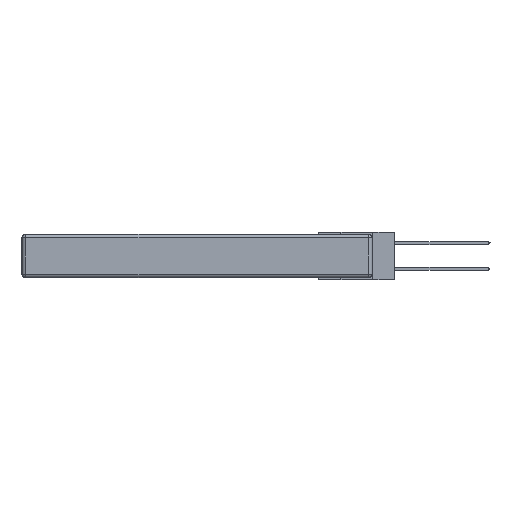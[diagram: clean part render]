
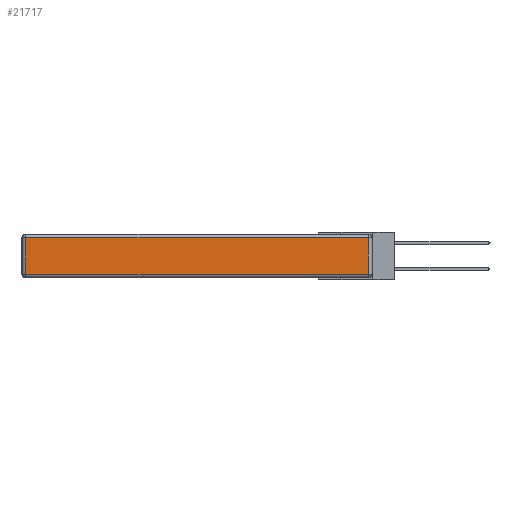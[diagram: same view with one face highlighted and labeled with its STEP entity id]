
A CAD part, left-side view. The second image highlights one B-rep face of the part: STEP entity #21717.
In plain terms, the highlighted planar face has unit normal (-1, 0, 0).
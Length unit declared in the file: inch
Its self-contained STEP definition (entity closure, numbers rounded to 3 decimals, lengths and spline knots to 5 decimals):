
#26 = DIRECTION ( 'NONE',  ( 0., 0., -1. ) ) ;
#100 = CARTESIAN_POINT ( 'NONE',  ( 0., 2.72, -0.313 ) ) ;
#958 = LINE ( 'NONE', #12153, #4760 ) ;
#1406 = ORIENTED_EDGE ( 'NONE', *, *, #11649, .T. ) ;
#1409 = LINE ( 'NONE', #20184, #4396 ) ;
#2361 = DIRECTION ( 'NONE',  ( -1., 0., 0. ) ) ;
#3458 = VERTEX_POINT ( 'NONE', #18017 ) ;
#4396 = VECTOR ( 'NONE', #4519, 39.37008 ) ;
#4519 = DIRECTION ( 'NONE',  ( 0., 1., 0. ) ) ;
#4760 = VECTOR ( 'NONE', #26, 39.37008 ) ;
#5442 = ORIENTED_EDGE ( 'NONE', *, *, #7664, .T. ) ;
#7530 = PLANE ( 'NONE',  #11340 ) ;
#7664 = EDGE_CURVE ( 'NONE', #20196, #15308, #10253, .T. ) ;
#8063 = CARTESIAN_POINT ( 'NONE',  ( 0., 0.03, -0.343 ) ) ;
#9069 = VERTEX_POINT ( 'NONE', #19718 ) ;
#9479 = EDGE_CURVE ( 'NONE', #9069, #20196, #958, .T. ) ;
#10253 = LINE ( 'NONE', #10655, #14064 ) ;
#10655 = CARTESIAN_POINT ( 'NONE',  ( 0., 0., -0.313 ) ) ;
#11340 = AXIS2_PLACEMENT_3D ( 'NONE', #19544, #2361, #18087 ) ;
#11627 = ORIENTED_EDGE ( 'NONE', *, *, #9479, .T. ) ;
#11649 = EDGE_CURVE ( 'NONE', #3458, #9069, #1409, .T. ) ;
#12153 = CARTESIAN_POINT ( 'NONE',  ( 0., 2.72, -0.343 ) ) ;
#14064 = VECTOR ( 'NONE', #17601, 39.37008 ) ;
#14900 = EDGE_LOOP ( 'NONE', ( #5442, #19117, #1406, #11627 ) ) ;
#15308 = VERTEX_POINT ( 'NONE', #21582 ) ;
#15827 = VECTOR ( 'NONE', #22045, 39.37008 ) ;
#17601 = DIRECTION ( 'NONE',  ( 0., -1., 0. ) ) ;
#18017 = CARTESIAN_POINT ( 'NONE',  ( 0., 0.03, -0.03 ) ) ;
#18087 = DIRECTION ( 'NONE',  ( 0., 0., 1. ) ) ;
#19117 = ORIENTED_EDGE ( 'NONE', *, *, #21583, .T. ) ;
#19544 = CARTESIAN_POINT ( 'NONE',  ( 0., 0., -0.343 ) ) ;
#19718 = CARTESIAN_POINT ( 'NONE',  ( 0., 2.72, -0.03 ) ) ;
#20184 = CARTESIAN_POINT ( 'NONE',  ( 0., 2.75, -0.03 ) ) ;
#20196 = VERTEX_POINT ( 'NONE', #100 ) ;
#21031 = LINE ( 'NONE', #8063, #15827 ) ;
#21294 = FACE_OUTER_BOUND ( 'NONE', #14900, .T. ) ;
#21582 = CARTESIAN_POINT ( 'NONE',  ( 0., 0.03, -0.313 ) ) ;
#21583 = EDGE_CURVE ( 'NONE', #15308, #3458, #21031, .T. ) ;
#21717 = ADVANCED_FACE ( 'NONE', ( #21294 ), #7530, .T. ) ;
#22045 = DIRECTION ( 'NONE',  ( 0., 0., 1. ) ) ;
